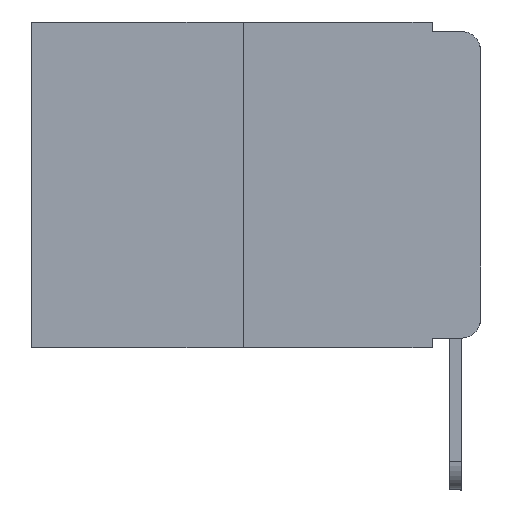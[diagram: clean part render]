
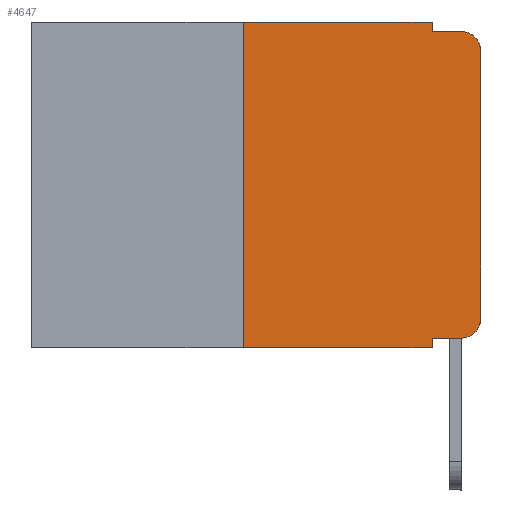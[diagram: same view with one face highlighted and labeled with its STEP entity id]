
A CAD part, left-side view. The second image highlights one B-rep face of the part: STEP entity #4647.
In plain terms, the highlighted planar face has unit normal (-1, 0, 0).
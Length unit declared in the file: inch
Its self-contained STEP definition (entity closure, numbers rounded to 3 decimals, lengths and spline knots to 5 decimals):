
#156 = DIRECTION ( 'NONE',  ( 1., 0., 0. ) ) ;
#285 = CARTESIAN_POINT ( 'NONE',  ( 0., 0.051, -0.333 ) ) ;
#302 = LINE ( 'NONE', #8937, #14438 ) ;
#434 = EDGE_CURVE ( 'NONE', #4187, #15779, #4555, .T. ) ;
#596 = CARTESIAN_POINT ( 'NONE',  ( 0., 0., -0.313 ) ) ;
#682 = VERTEX_POINT ( 'NONE', #9646 ) ;
#929 = DIRECTION ( 'NONE',  ( 0., 0., -1. ) ) ;
#1189 = ORIENTED_EDGE ( 'NONE', *, *, #8860, .F. ) ;
#1571 = ORIENTED_EDGE ( 'NONE', *, *, #13234, .F. ) ;
#1942 = VECTOR ( 'NONE', #13724, 39.37008 ) ;
#2105 = ORIENTED_EDGE ( 'NONE', *, *, #10081, .T. ) ;
#2222 = CARTESIAN_POINT ( 'NONE',  ( 0., 0.051, -0.01 ) ) ;
#3557 = AXIS2_PLACEMENT_3D ( 'NONE', #11799, #13457, #16249 ) ;
#3683 = DIRECTION ( 'NONE',  ( 0., 0., -1. ) ) ;
#3736 = CARTESIAN_POINT ( 'NONE',  ( 0., 0.02, -0.333 ) ) ;
#3914 = EDGE_LOOP ( 'NONE', ( #2105, #15740, #1571, #15246, #7660, #17434, #8979, #1189, #12719, #7547 ) ) ;
#4015 = VECTOR ( 'NONE', #15280, 39.37008 ) ;
#4187 = VERTEX_POINT ( 'NONE', #12902 ) ;
#4555 = LINE ( 'NONE', #285, #16255 ) ;
#4647 = ADVANCED_FACE ( 'NONE', ( #15563 ), #14088, .F. ) ;
#6052 = VECTOR ( 'NONE', #929, 39.37008 ) ;
#6994 = CARTESIAN_POINT ( 'NONE',  ( 0., 0.02, -0.01 ) ) ;
#7296 = LINE ( 'NONE', #15648, #12628 ) ;
#7394 = LINE ( 'NONE', #11494, #14549 ) ;
#7468 = CARTESIAN_POINT ( 'NONE',  ( 0., 0.051, -0.01 ) ) ;
#7547 = ORIENTED_EDGE ( 'NONE', *, *, #16208, .T. ) ;
#7660 = ORIENTED_EDGE ( 'NONE', *, *, #10875, .F. ) ;
#8131 = DIRECTION ( 'NONE',  ( -1., 0., 0. ) ) ;
#8176 = EDGE_CURVE ( 'NONE', #11481, #16289, #18331, .T. ) ;
#8190 = VECTOR ( 'NONE', #15127, 39.37008 ) ;
#8860 = EDGE_CURVE ( 'NONE', #4187, #16289, #16418, .T. ) ;
#8937 = CARTESIAN_POINT ( 'NONE',  ( 0., 0., 0. ) ) ;
#8979 = ORIENTED_EDGE ( 'NONE', *, *, #8176, .T. ) ;
#9311 = EDGE_CURVE ( 'NONE', #682, #14267, #17374, .T. ) ;
#9461 = LINE ( 'NONE', #2222, #8190 ) ;
#9588 = VERTEX_POINT ( 'NONE', #596 ) ;
#9609 = CARTESIAN_POINT ( 'NONE',  ( 0., 0.02, -0.03 ) ) ;
#9646 = CARTESIAN_POINT ( 'NONE',  ( 0., 0., -0.03 ) ) ;
#10081 = EDGE_CURVE ( 'NONE', #9588, #682, #302, .T. ) ;
#10183 = DIRECTION ( 'NONE',  ( 0., 0., 1. ) ) ;
#10224 = DIRECTION ( 'NONE',  ( 0., -1., 0. ) ) ;
#10484 = CARTESIAN_POINT ( 'NONE',  ( 0., 0.051, -0.343 ) ) ;
#10787 = CARTESIAN_POINT ( 'NONE',  ( 0., 0.25, -0.343 ) ) ;
#10875 = EDGE_CURVE ( 'NONE', #11154, #15005, #7296, .T. ) ;
#11154 = VERTEX_POINT ( 'NONE', #16479 ) ;
#11216 = CARTESIAN_POINT ( 'NONE',  ( 0., 0.473, 0. ) ) ;
#11481 = VERTEX_POINT ( 'NONE', #10787 ) ;
#11494 = CARTESIAN_POINT ( 'NONE',  ( 0., 0.25, 0. ) ) ;
#11799 = CARTESIAN_POINT ( 'NONE',  ( 0., 0.02, -0.313 ) ) ;
#11945 = EDGE_CURVE ( 'NONE', #15005, #15302, #13732, .T. ) ;
#12628 = VECTOR ( 'NONE', #15546, 39.37008 ) ;
#12719 = ORIENTED_EDGE ( 'NONE', *, *, #434, .T. ) ;
#12751 = CIRCLE ( 'NONE', #3557, 0.02 ) ;
#12902 = CARTESIAN_POINT ( 'NONE',  ( 0., 0.051, -0.333 ) ) ;
#13234 = EDGE_CURVE ( 'NONE', #15302, #14267, #9461, .T. ) ;
#13457 = DIRECTION ( 'NONE',  ( -1., 0., 0. ) ) ;
#13552 = CARTESIAN_POINT ( 'NONE',  ( 0., 0.051, 0. ) ) ;
#13724 = DIRECTION ( 'NONE',  ( 0., 0., -1. ) ) ;
#13732 = LINE ( 'NONE', #14764, #6052 ) ;
#14088 = PLANE ( 'NONE',  #14458 ) ;
#14135 = AXIS2_PLACEMENT_3D ( 'NONE', #9609, #8131, #3683 ) ;
#14167 = CARTESIAN_POINT ( 'NONE',  ( 0., 0.473, -0.343 ) ) ;
#14267 = VERTEX_POINT ( 'NONE', #6994 ) ;
#14438 = VECTOR ( 'NONE', #17475, 39.37008 ) ;
#14458 = AXIS2_PLACEMENT_3D ( 'NONE', #11216, #156, #15749 ) ;
#14549 = VECTOR ( 'NONE', #10183, 39.37008 ) ;
#14764 = CARTESIAN_POINT ( 'NONE',  ( 0., 0.051, 0. ) ) ;
#15005 = VERTEX_POINT ( 'NONE', #15192 ) ;
#15127 = DIRECTION ( 'NONE',  ( 0., -1., 0. ) ) ;
#15192 = CARTESIAN_POINT ( 'NONE',  ( 0., 0.051, 0. ) ) ;
#15246 = ORIENTED_EDGE ( 'NONE', *, *, #11945, .F. ) ;
#15280 = DIRECTION ( 'NONE',  ( 0., -1., 0. ) ) ;
#15302 = VERTEX_POINT ( 'NONE', #7468 ) ;
#15546 = DIRECTION ( 'NONE',  ( 0., -1., 0. ) ) ;
#15563 = FACE_OUTER_BOUND ( 'NONE', #3914, .T. ) ;
#15648 = CARTESIAN_POINT ( 'NONE',  ( 0., 0.473, 0. ) ) ;
#15740 = ORIENTED_EDGE ( 'NONE', *, *, #9311, .T. ) ;
#15749 = DIRECTION ( 'NONE',  ( 0., 0., -1. ) ) ;
#15779 = VERTEX_POINT ( 'NONE', #3736 ) ;
#16208 = EDGE_CURVE ( 'NONE', #15779, #9588, #12751, .T. ) ;
#16249 = DIRECTION ( 'NONE',  ( 0., 0., -1. ) ) ;
#16255 = VECTOR ( 'NONE', #10224, 39.37008 ) ;
#16289 = VERTEX_POINT ( 'NONE', #10484 ) ;
#16418 = LINE ( 'NONE', #13552, #1942 ) ;
#16479 = CARTESIAN_POINT ( 'NONE',  ( 0., 0.25, 0. ) ) ;
#16934 = EDGE_CURVE ( 'NONE', #11481, #11154, #7394, .T. ) ;
#17374 = CIRCLE ( 'NONE', #14135, 0.02 ) ;
#17434 = ORIENTED_EDGE ( 'NONE', *, *, #16934, .F. ) ;
#17475 = DIRECTION ( 'NONE',  ( 0., 0., 1. ) ) ;
#18331 = LINE ( 'NONE', #14167, #4015 ) ;
